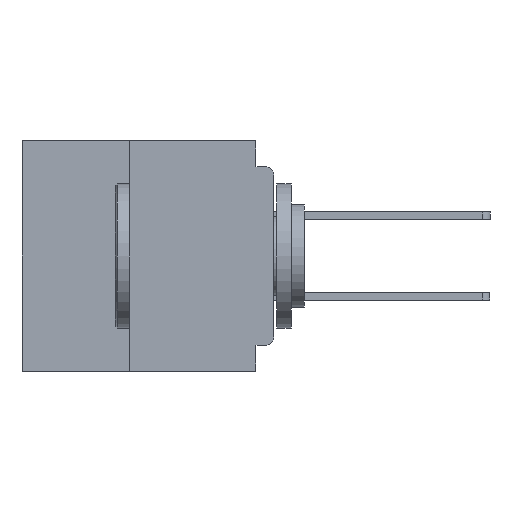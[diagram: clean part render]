
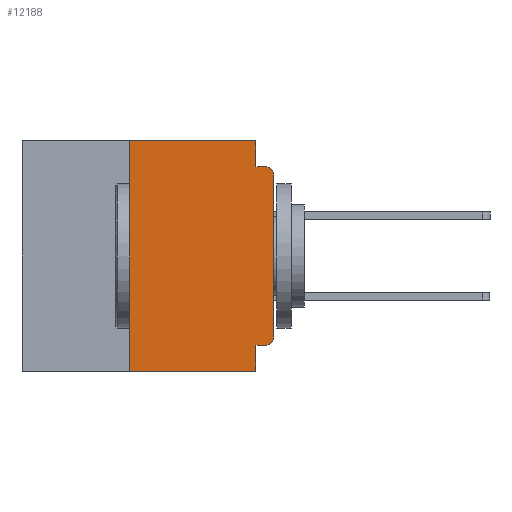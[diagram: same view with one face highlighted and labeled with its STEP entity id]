
A CAD part, left-side view. The second image highlights one B-rep face of the part: STEP entity #12188.
In plain terms, the highlighted planar face has unit normal (-1, 0, 0).
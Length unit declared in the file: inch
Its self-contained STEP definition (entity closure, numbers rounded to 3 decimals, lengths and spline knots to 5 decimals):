
#338 = ORIENTED_EDGE ( 'NONE', *, *, #26765, .F. ) ;
#1475 = LINE ( 'NONE', #35838, #30716 ) ;
#1531 = CARTESIAN_POINT ( 'NONE',  ( 0., 0., -0.06 ) ) ;
#2127 = CIRCLE ( 'NONE', #16532, 0.015 ) ;
#2713 = DIRECTION ( 'NONE',  ( 0., -1., 0. ) ) ;
#2848 = VERTEX_POINT ( 'NONE', #37910 ) ;
#3251 = VECTOR ( 'NONE', #9909, 39.37008 ) ;
#4007 = ORIENTED_EDGE ( 'NONE', *, *, #21324, .T. ) ;
#4262 = LINE ( 'NONE', #25170, #38743 ) ;
#4569 = ORIENTED_EDGE ( 'NONE', *, *, #14741, .F. ) ;
#6107 = ORIENTED_EDGE ( 'NONE', *, *, #14847, .F. ) ;
#6230 = AXIS2_PLACEMENT_3D ( 'NONE', #16731, #40099, #20035 ) ;
#7685 = ORIENTED_EDGE ( 'NONE', *, *, #39667, .T. ) ;
#8250 = VERTEX_POINT ( 'NONE', #33524 ) ;
#9357 = CARTESIAN_POINT ( 'NONE',  ( 0., 0.437, 0. ) ) ;
#9909 = DIRECTION ( 'NONE',  ( 0., 0., 1. ) ) ;
#10309 = ORIENTED_EDGE ( 'NONE', *, *, #12434, .F. ) ;
#10571 = VERTEX_POINT ( 'NONE', #38886 ) ;
#11078 = PLANE ( 'NONE',  #12265 ) ;
#11127 = LINE ( 'NONE', #39818, #3251 ) ;
#12188 = ADVANCED_FACE ( 'NONE', ( #23392 ), #11078, .F. ) ;
#12265 = AXIS2_PLACEMENT_3D ( 'NONE', #31061, #14425, #37778 ) ;
#12423 = ORIENTED_EDGE ( 'NONE', *, *, #40153, .T. ) ;
#12434 = EDGE_CURVE ( 'NONE', #19329, #12910, #1475, .T. ) ;
#12910 = VERTEX_POINT ( 'NONE', #14799 ) ;
#14178 = VERTEX_POINT ( 'NONE', #42339 ) ;
#14372 = VERTEX_POINT ( 'NONE', #30226 ) ;
#14425 = DIRECTION ( 'NONE',  ( 1., 0., 0. ) ) ;
#14741 = EDGE_CURVE ( 'NONE', #18929, #19329, #30493, .T. ) ;
#14799 = CARTESIAN_POINT ( 'NONE',  ( 0., 0.031, -0.045 ) ) ;
#14847 = EDGE_CURVE ( 'NONE', #14178, #21091, #26248, .T. ) ;
#15695 = DIRECTION ( 'NONE',  ( -1., 0., 0. ) ) ;
#15852 = DIRECTION ( 'NONE',  ( 0., -1., 0. ) ) ;
#16532 = AXIS2_PLACEMENT_3D ( 'NONE', #35676, #15695, #39049 ) ;
#16731 = CARTESIAN_POINT ( 'NONE',  ( 0., 0.015, -0.06 ) ) ;
#17304 = EDGE_CURVE ( 'NONE', #24042, #14372, #32946, .T. ) ;
#17413 = VECTOR ( 'NONE', #40123, 39.37008 ) ;
#18929 = VERTEX_POINT ( 'NONE', #26040 ) ;
#19329 = VERTEX_POINT ( 'NONE', #29007 ) ;
#20035 = DIRECTION ( 'NONE',  ( 0., 0., -1. ) ) ;
#21091 = VERTEX_POINT ( 'NONE', #42154 ) ;
#21118 = EDGE_CURVE ( 'NONE', #2848, #18929, #28338, .T. ) ;
#21324 = EDGE_CURVE ( 'NONE', #10571, #24042, #11127, .T. ) ;
#21595 = VECTOR ( 'NONE', #32689, 39.37008 ) ;
#22287 = ORIENTED_EDGE ( 'NONE', *, *, #21118, .F. ) ;
#22697 = CARTESIAN_POINT ( 'NONE',  ( 0., 0., -0.045 ) ) ;
#22782 = ORIENTED_EDGE ( 'NONE', *, *, #17304, .T. ) ;
#23392 = FACE_OUTER_BOUND ( 'NONE', #26724, .T. ) ;
#24042 = VERTEX_POINT ( 'NONE', #1531 ) ;
#24961 = LINE ( 'NONE', #22697, #42728 ) ;
#25049 = EDGE_CURVE ( 'NONE', #8250, #14178, #38733, .T. ) ;
#25170 = CARTESIAN_POINT ( 'NONE',  ( 0., 0.437, -0.4 ) ) ;
#26040 = CARTESIAN_POINT ( 'NONE',  ( 0., 0.25, 0. ) ) ;
#26248 = LINE ( 'NONE', #36749, #17413 ) ;
#26724 = EDGE_LOOP ( 'NONE', ( #4007, #22782, #338, #10309, #4569, #22287, #7685, #6107, #26948, #12423 ) ) ;
#26765 = EDGE_CURVE ( 'NONE', #12910, #14372, #24961, .T. ) ;
#26801 = DIRECTION ( 'NONE',  ( 0., 1., 0. ) ) ;
#26948 = ORIENTED_EDGE ( 'NONE', *, *, #25049, .F. ) ;
#27267 = VECTOR ( 'NONE', #38953, 39.37008 ) ;
#28338 = LINE ( 'NONE', #35444, #27267 ) ;
#29007 = CARTESIAN_POINT ( 'NONE',  ( 0., 0.031, 0. ) ) ;
#29851 = VECTOR ( 'NONE', #26801, 39.37008 ) ;
#30226 = CARTESIAN_POINT ( 'NONE',  ( 0., 0.015, -0.045 ) ) ;
#30493 = LINE ( 'NONE', #9357, #21595 ) ;
#30716 = VECTOR ( 'NONE', #32514, 39.37008 ) ;
#31061 = CARTESIAN_POINT ( 'NONE',  ( 0., 0.437, 0. ) ) ;
#32514 = DIRECTION ( 'NONE',  ( 0., 0., -1. ) ) ;
#32689 = DIRECTION ( 'NONE',  ( 0., -1., 0. ) ) ;
#32946 = CIRCLE ( 'NONE', #6230, 0.015 ) ;
#33401 = CARTESIAN_POINT ( 'NONE',  ( 0., 0., -0.355 ) ) ;
#33524 = CARTESIAN_POINT ( 'NONE',  ( 0., 0.015, -0.355 ) ) ;
#35444 = CARTESIAN_POINT ( 'NONE',  ( 0., 0.25, -0.4 ) ) ;
#35676 = CARTESIAN_POINT ( 'NONE',  ( 0., 0.015, -0.34 ) ) ;
#35838 = CARTESIAN_POINT ( 'NONE',  ( 0., 0.031, 0. ) ) ;
#36749 = CARTESIAN_POINT ( 'NONE',  ( 0., 0.031, -0.4 ) ) ;
#37778 = DIRECTION ( 'NONE',  ( 0., 0., -1. ) ) ;
#37910 = CARTESIAN_POINT ( 'NONE',  ( 0., 0.25, -0.4 ) ) ;
#38733 = LINE ( 'NONE', #33401, #29851 ) ;
#38743 = VECTOR ( 'NONE', #15852, 39.37008 ) ;
#38886 = CARTESIAN_POINT ( 'NONE',  ( 0., 0., -0.34 ) ) ;
#38953 = DIRECTION ( 'NONE',  ( 0., 0., 1. ) ) ;
#39049 = DIRECTION ( 'NONE',  ( 0., 0., -1. ) ) ;
#39667 = EDGE_CURVE ( 'NONE', #2848, #21091, #4262, .T. ) ;
#39818 = CARTESIAN_POINT ( 'NONE',  ( 0., 0., 0. ) ) ;
#40099 = DIRECTION ( 'NONE',  ( -1., 0., 0. ) ) ;
#40123 = DIRECTION ( 'NONE',  ( 0., 0., -1. ) ) ;
#40153 = EDGE_CURVE ( 'NONE', #8250, #10571, #2127, .T. ) ;
#42154 = CARTESIAN_POINT ( 'NONE',  ( 0., 0.031, -0.4 ) ) ;
#42339 = CARTESIAN_POINT ( 'NONE',  ( 0., 0.031, -0.355 ) ) ;
#42728 = VECTOR ( 'NONE', #2713, 39.37008 ) ;
